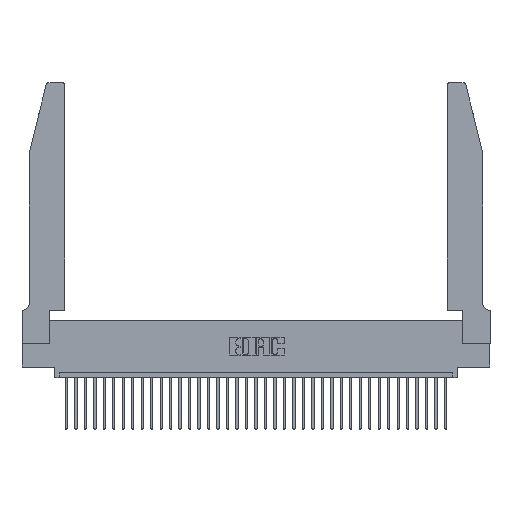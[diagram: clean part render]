
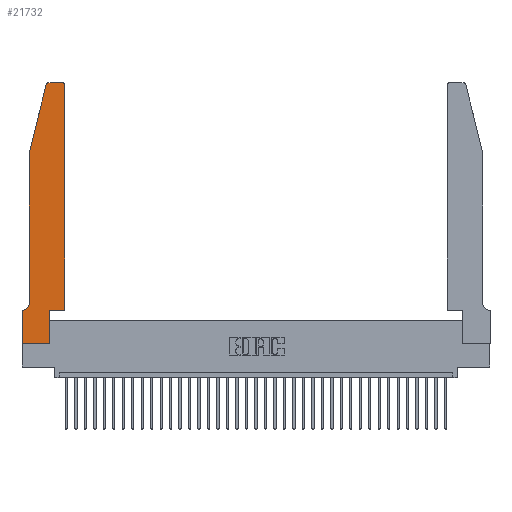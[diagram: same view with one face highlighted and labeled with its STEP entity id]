
A CAD part, top view. The second image highlights one B-rep face of the part: STEP entity #21732.
In plain terms, the highlighted planar face has unit normal (0, 0, 1).
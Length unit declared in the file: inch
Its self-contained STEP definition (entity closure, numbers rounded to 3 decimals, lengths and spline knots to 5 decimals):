
#390 = EDGE_CURVE ( 'NONE', #30356, #5047, #4404, .T. ) ;
#671 = DIRECTION ( 'NONE',  ( 0., -1., 0. ) ) ;
#725 = ORIENTED_EDGE ( 'NONE', *, *, #13415, .T. ) ;
#775 = PLANE ( 'NONE',  #5271 ) ;
#942 = ORIENTED_EDGE ( 'NONE', *, *, #29268, .T. ) ;
#2091 = EDGE_CURVE ( 'NONE', #25654, #31121, #29519, .T. ) ;
#2181 = CARTESIAN_POINT ( 'NONE',  ( 0.2865, 0.35, 0.37 ) ) ;
#2315 = CARTESIAN_POINT ( 'NONE',  ( 0.0755, 2., 0.37 ) ) ;
#2713 = DIRECTION ( 'NONE',  ( 0., 0., 1. ) ) ;
#2813 = DIRECTION ( 'NONE',  ( 0., 1., 0. ) ) ;
#3360 = VECTOR ( 'NONE', #671, 39.37008 ) ;
#3709 = CARTESIAN_POINT ( 'NONE',  ( 0.4205, 2.75, 0.37 ) ) ;
#3940 = LINE ( 'NONE', #31565, #20365 ) ;
#3941 = CARTESIAN_POINT ( 'NONE',  ( 0.2865, 0., 0.37 ) ) ;
#4404 = LINE ( 'NONE', #9187, #29926 ) ;
#4854 = VECTOR ( 'NONE', #2813, 39.37008 ) ;
#5035 = DIRECTION ( 'NONE',  ( -0.239, -0.971, 0. ) ) ;
#5047 = VERTEX_POINT ( 'NONE', #11104 ) ;
#5087 = VERTEX_POINT ( 'NONE', #14131 ) ;
#5246 = CARTESIAN_POINT ( 'NONE',  ( 0.4205, 2.72, 0.37 ) ) ;
#5271 = AXIS2_PLACEMENT_3D ( 'NONE', #31263, #22915, #25614 ) ;
#5430 = AXIS2_PLACEMENT_3D ( 'NONE', #5246, #19107, #19338 ) ;
#5632 = CARTESIAN_POINT ( 'NONE',  ( 0.284, 2.72, 0.37 ) ) ;
#6009 = VECTOR ( 'NONE', #33825, 39.37008 ) ;
#6442 = CIRCLE ( 'NONE', #5430, 0.03 ) ;
#6994 = EDGE_LOOP ( 'NONE', ( #32853, #16910, #725, #12646, #942, #33476, #28275, #9623, #18654, #22393, #31759, #29741 ) ) ;
#7306 = CIRCLE ( 'NONE', #12938, 0.03 ) ;
#8157 = VERTEX_POINT ( 'NONE', #16279 ) ;
#8188 = CARTESIAN_POINT ( 'NONE',  ( 0., 0., 0.37 ) ) ;
#8515 = DIRECTION ( 'NONE',  ( 1., 0., 0. ) ) ;
#8681 = CIRCLE ( 'NONE', #30429, 0.07 ) ;
#9187 = CARTESIAN_POINT ( 'NONE',  ( 0.2605, 2.75, 0.37 ) ) ;
#9623 = ORIENTED_EDGE ( 'NONE', *, *, #33884, .T. ) ;
#10231 = CARTESIAN_POINT ( 'NONE',  ( 0.0055, 0.42, 0.37 ) ) ;
#10633 = CARTESIAN_POINT ( 'NONE',  ( 0.4505, 0.35, 0.37 ) ) ;
#11104 = CARTESIAN_POINT ( 'NONE',  ( 0.284, 2.75, 0.37 ) ) ;
#11289 = VERTEX_POINT ( 'NONE', #20299 ) ;
#11578 = FACE_OUTER_BOUND ( 'NONE', #6994, .T. ) ;
#11771 = EDGE_CURVE ( 'NONE', #28064, #5087, #32371, .T. ) ;
#12646 = ORIENTED_EDGE ( 'NONE', *, *, #11771, .T. ) ;
#12800 = DIRECTION ( 'NONE',  ( 0., 1., 0. ) ) ;
#12938 = AXIS2_PLACEMENT_3D ( 'NONE', #5632, #2713, #8515 ) ;
#13415 = EDGE_CURVE ( 'NONE', #16971, #28064, #24871, .T. ) ;
#13721 = CARTESIAN_POINT ( 'NONE',  ( 0., 0., 0.37 ) ) ;
#14131 = CARTESIAN_POINT ( 'NONE',  ( 0.0755, 0.42, 0.37 ) ) ;
#14865 = CARTESIAN_POINT ( 'NONE',  ( 0.4505, 0.35, 0.37 ) ) ;
#16279 = CARTESIAN_POINT ( 'NONE',  ( 0., 0.35, 0.37 ) ) ;
#16587 = VERTEX_POINT ( 'NONE', #3941 ) ;
#16910 = ORIENTED_EDGE ( 'NONE', *, *, #33790, .T. ) ;
#16971 = VERTEX_POINT ( 'NONE', #24210 ) ;
#17365 = CARTESIAN_POINT ( 'NONE',  ( 0.0755, 2., 0.37 ) ) ;
#17530 = CARTESIAN_POINT ( 'NONE',  ( 0.2865, 0.35, 0.37 ) ) ;
#17632 = DIRECTION ( 'NONE',  ( -1., 0., 0. ) ) ;
#17720 = DIRECTION ( 'NONE',  ( -1., 0., 0. ) ) ;
#17772 = EDGE_CURVE ( 'NONE', #8157, #26604, #32251, .T. ) ;
#17986 = DIRECTION ( 'NONE',  ( -1., 0., 0. ) ) ;
#18648 = CARTESIAN_POINT ( 'NONE',  ( 0.0755, 2., 0.37 ) ) ;
#18654 = ORIENTED_EDGE ( 'NONE', *, *, #27756, .T. ) ;
#19107 = DIRECTION ( 'NONE',  ( 0., 0., 1. ) ) ;
#19338 = DIRECTION ( 'NONE',  ( 1., 0., 0. ) ) ;
#19739 = CARTESIAN_POINT ( 'NONE',  ( 0., 0., 0.37 ) ) ;
#20299 = CARTESIAN_POINT ( 'NONE',  ( 0.0055, 0.35, 0.37 ) ) ;
#20365 = VECTOR ( 'NONE', #34385, 39.37008 ) ;
#20830 = EDGE_CURVE ( 'NONE', #22879, #25654, #3940, .T. ) ;
#21502 = LINE ( 'NONE', #23195, #22339 ) ;
#21732 = ADVANCED_FACE ( 'NONE', ( #11578 ), #775, .T. ) ;
#22339 = VECTOR ( 'NONE', #17720, 39.37008 ) ;
#22393 = ORIENTED_EDGE ( 'NONE', *, *, #20830, .T. ) ;
#22879 = VERTEX_POINT ( 'NONE', #17530 ) ;
#22915 = DIRECTION ( 'NONE',  ( 0., 0., 1. ) ) ;
#23195 = CARTESIAN_POINT ( 'NONE',  ( 0.0755, 0.35, 0.37 ) ) ;
#23305 = LINE ( 'NONE', #19739, #6009 ) ;
#23567 = VECTOR ( 'NONE', #31288, 39.37008 ) ;
#24210 = CARTESIAN_POINT ( 'NONE',  ( 0.25487, 2.72718, 0.37 ) ) ;
#24871 = LINE ( 'NONE', #18648, #25755 ) ;
#25614 = DIRECTION ( 'NONE',  ( 1., 0., 0. ) ) ;
#25654 = VERTEX_POINT ( 'NONE', #14865 ) ;
#25755 = VECTOR ( 'NONE', #5035, 39.37008 ) ;
#26604 = VERTEX_POINT ( 'NONE', #8188 ) ;
#27756 = EDGE_CURVE ( 'NONE', #16587, #22879, #27894, .T. ) ;
#27894 = LINE ( 'NONE', #2181, #34380 ) ;
#28064 = VERTEX_POINT ( 'NONE', #17365 ) ;
#28275 = ORIENTED_EDGE ( 'NONE', *, *, #17772, .T. ) ;
#29268 = EDGE_CURVE ( 'NONE', #5087, #11289, #8681, .T. ) ;
#29519 = LINE ( 'NONE', #10633, #4854 ) ;
#29628 = DIRECTION ( 'NONE',  ( 0., 0., -1. ) ) ;
#29741 = ORIENTED_EDGE ( 'NONE', *, *, #30741, .T. ) ;
#29926 = VECTOR ( 'NONE', #17632, 39.37008 ) ;
#30356 = VERTEX_POINT ( 'NONE', #3709 ) ;
#30429 = AXIS2_PLACEMENT_3D ( 'NONE', #10231, #29628, #17986 ) ;
#30741 = EDGE_CURVE ( 'NONE', #31121, #30356, #6442, .T. ) ;
#31121 = VERTEX_POINT ( 'NONE', #32042 ) ;
#31263 = CARTESIAN_POINT ( 'NONE',  ( 0., 0.35, 0.37 ) ) ;
#31288 = DIRECTION ( 'NONE',  ( 0., -1., 0. ) ) ;
#31565 = CARTESIAN_POINT ( 'NONE',  ( 0.4505, 0.35, 0.37 ) ) ;
#31759 = ORIENTED_EDGE ( 'NONE', *, *, #2091, .T. ) ;
#32042 = CARTESIAN_POINT ( 'NONE',  ( 0.4505, 2.72, 0.37 ) ) ;
#32251 = LINE ( 'NONE', #13721, #23567 ) ;
#32371 = LINE ( 'NONE', #2315, #3360 ) ;
#32853 = ORIENTED_EDGE ( 'NONE', *, *, #390, .T. ) ;
#33476 = ORIENTED_EDGE ( 'NONE', *, *, #34973, .T. ) ;
#33790 = EDGE_CURVE ( 'NONE', #5047, #16971, #7306, .T. ) ;
#33825 = DIRECTION ( 'NONE',  ( 1., 0., 0. ) ) ;
#33884 = EDGE_CURVE ( 'NONE', #26604, #16587, #23305, .T. ) ;
#34380 = VECTOR ( 'NONE', #12800, 39.37008 ) ;
#34385 = DIRECTION ( 'NONE',  ( 1., 0., 0. ) ) ;
#34973 = EDGE_CURVE ( 'NONE', #11289, #8157, #21502, .T. ) ;
